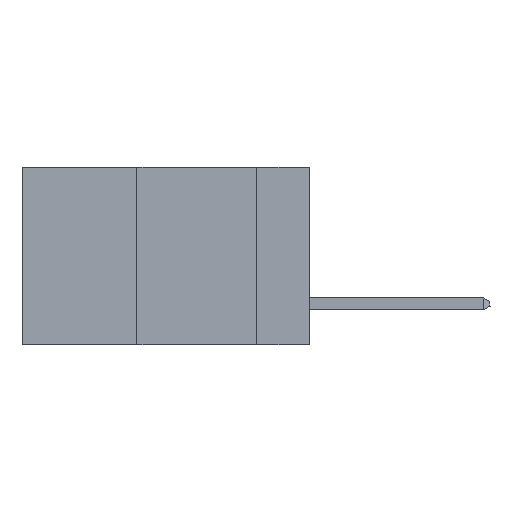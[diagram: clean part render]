
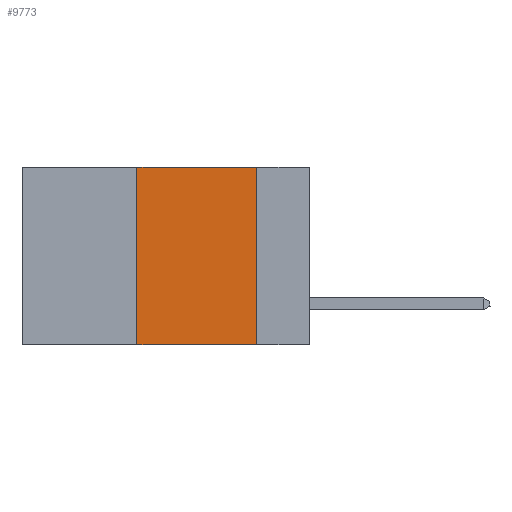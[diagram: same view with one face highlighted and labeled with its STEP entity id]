
A CAD part, left-side view. The second image highlights one B-rep face of the part: STEP entity #9773.
In plain terms, the highlighted planar face has unit normal (-1, 0, 0).
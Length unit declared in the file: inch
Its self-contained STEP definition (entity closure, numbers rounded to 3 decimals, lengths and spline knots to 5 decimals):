
#489 = CARTESIAN_POINT ( 'NONE',  ( 0., 0.36, 0. ) ) ;
#542 = VERTEX_POINT ( 'NONE', #9781 ) ;
#1136 = LINE ( 'NONE', #3828, #1851 ) ;
#1347 = CARTESIAN_POINT ( 'NONE',  ( 0., 0.6, 0. ) ) ;
#1687 = EDGE_CURVE ( 'NONE', #542, #2002, #9802, .T. ) ;
#1851 = VECTOR ( 'NONE', #9053, 39.37008 ) ;
#1978 = VECTOR ( 'NONE', #9840, 39.37008 ) ;
#2002 = VERTEX_POINT ( 'NONE', #9682 ) ;
#2945 = ORIENTED_EDGE ( 'NONE', *, *, #5967, .F. ) ;
#3099 = CARTESIAN_POINT ( 'NONE',  ( 0., 0.6, -0.37 ) ) ;
#3491 = CARTESIAN_POINT ( 'NONE',  ( 0., 0.36, 0. ) ) ;
#3792 = ORIENTED_EDGE ( 'NONE', *, *, #5509, .F. ) ;
#3828 = CARTESIAN_POINT ( 'NONE',  ( 0., 0.6, 0. ) ) ;
#4152 = PLANE ( 'NONE',  #11596 ) ;
#5509 = EDGE_CURVE ( 'NONE', #7579, #2002, #10123, .T. ) ;
#5853 = DIRECTION ( 'NONE',  ( 0., -1., 0. ) ) ;
#5967 = EDGE_CURVE ( 'NONE', #10101, #7579, #1136, .T. ) ;
#6209 = DIRECTION ( 'NONE',  ( 0., 0., 1. ) ) ;
#7068 = CARTESIAN_POINT ( 'NONE',  ( 0., 0.11, 0. ) ) ;
#7188 = EDGE_LOOP ( 'NONE', ( #3792, #2945, #9701, #7489 ) ) ;
#7264 = FACE_OUTER_BOUND ( 'NONE', #7188, .T. ) ;
#7326 = VECTOR ( 'NONE', #5853, 39.37008 ) ;
#7489 = ORIENTED_EDGE ( 'NONE', *, *, #1687, .T. ) ;
#7579 = VERTEX_POINT ( 'NONE', #7068 ) ;
#7614 = LINE ( 'NONE', #489, #8050 ) ;
#7620 = EDGE_CURVE ( 'NONE', #542, #10101, #7614, .T. ) ;
#7692 = DIRECTION ( 'NONE',  ( 0., 0., -1. ) ) ;
#8050 = VECTOR ( 'NONE', #6209, 39.37008 ) ;
#8907 = CARTESIAN_POINT ( 'NONE',  ( 0., 0.11, 0. ) ) ;
#9053 = DIRECTION ( 'NONE',  ( 0., -1., 0. ) ) ;
#9682 = CARTESIAN_POINT ( 'NONE',  ( 0., 0.11, -0.37 ) ) ;
#9701 = ORIENTED_EDGE ( 'NONE', *, *, #7620, .F. ) ;
#9773 = ADVANCED_FACE ( 'NONE', ( #7264 ), #4152, .F. ) ;
#9781 = CARTESIAN_POINT ( 'NONE',  ( 0., 0.36, -0.37 ) ) ;
#9802 = LINE ( 'NONE', #3099, #7326 ) ;
#9840 = DIRECTION ( 'NONE',  ( 0., 0., -1. ) ) ;
#10101 = VERTEX_POINT ( 'NONE', #3491 ) ;
#10123 = LINE ( 'NONE', #8907, #1978 ) ;
#10499 = DIRECTION ( 'NONE',  ( 1., 0., 0. ) ) ;
#11596 = AXIS2_PLACEMENT_3D ( 'NONE', #1347, #10499, #7692 ) ;
